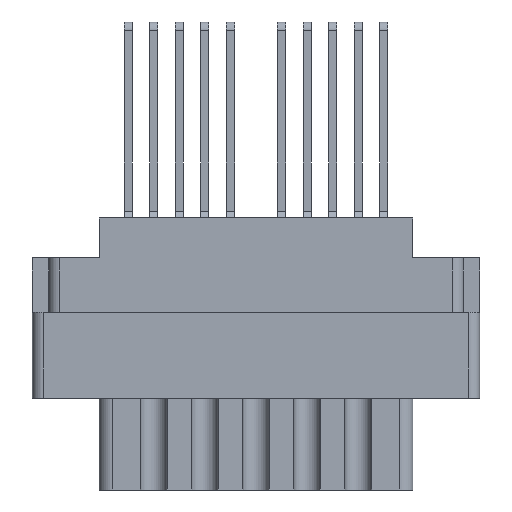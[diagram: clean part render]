
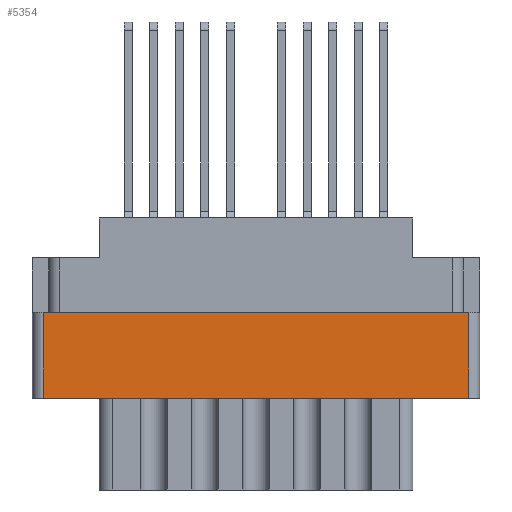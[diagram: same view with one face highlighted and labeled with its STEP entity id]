
A CAD part, front view. The second image highlights one B-rep face of the part: STEP entity #5354.
In plain terms, the highlighted planar face has unit normal (0, -1, 0).
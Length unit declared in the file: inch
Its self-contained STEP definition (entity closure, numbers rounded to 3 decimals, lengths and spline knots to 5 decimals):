
#2116 = VECTOR ( 'NONE', #2926, 39.37008 ) ;
#2384 = ORIENTED_EDGE ( 'NONE', *, *, #20708, .F. ) ;
#2432 = LINE ( 'NONE', #14155, #11054 ) ;
#2926 = DIRECTION ( 'NONE',  ( 1., 0., 0. ) ) ;
#2993 = CARTESIAN_POINT ( 'NONE',  ( -0.656, -0.343, -0.798 ) ) ;
#3983 = CARTESIAN_POINT ( 'NONE',  ( 0.624, -0.343, -0.277 ) ) ;
#5354 = ADVANCED_FACE ( 'NONE', ( #11126 ), #17944, .T. ) ;
#5846 = CARTESIAN_POINT ( 'NONE',  ( -0.624, -0.343, -0.798 ) ) ;
#7570 = ORIENTED_EDGE ( 'NONE', *, *, #15330, .F. ) ;
#8149 = VECTOR ( 'NONE', #13333, 39.37008 ) ;
#8384 = CARTESIAN_POINT ( 'NONE',  ( -0.624, -0.343, -0.529 ) ) ;
#11054 = VECTOR ( 'NONE', #14006, 39.37008 ) ;
#11126 = FACE_OUTER_BOUND ( 'NONE', #18625, .T. ) ;
#11154 = ORIENTED_EDGE ( 'NONE', *, *, #22824, .T. ) ;
#13168 = VECTOR ( 'NONE', #17793, 39.37008 ) ;
#13333 = DIRECTION ( 'NONE',  ( 0., 0., -1. ) ) ;
#13719 = LINE ( 'NONE', #5846, #8149 ) ;
#13905 = LINE ( 'NONE', #19345, #2116 ) ;
#13915 = VERTEX_POINT ( 'NONE', #3983 ) ;
#14006 = DIRECTION ( 'NONE',  ( -1., 0., 0. ) ) ;
#14082 = DIRECTION ( 'NONE',  ( 0., -1., 0. ) ) ;
#14155 = CARTESIAN_POINT ( 'NONE',  ( 0., -0.343, -0.529 ) ) ;
#14399 = CARTESIAN_POINT ( 'NONE',  ( 0.624, -0.343, -0.798 ) ) ;
#14487 = VERTEX_POINT ( 'NONE', #20200 ) ;
#15330 = EDGE_CURVE ( 'NONE', #22295, #13915, #13905, .T. ) ;
#16072 = DIRECTION ( 'NONE',  ( 0., 0., -1. ) ) ;
#16103 = CARTESIAN_POINT ( 'NONE',  ( -0.624, -0.343, -0.277 ) ) ;
#16345 = EDGE_CURVE ( 'NONE', #22295, #19529, #13719, .T. ) ;
#17549 = ORIENTED_EDGE ( 'NONE', *, *, #16345, .T. ) ;
#17793 = DIRECTION ( 'NONE',  ( 0., 0., 1. ) ) ;
#17944 = PLANE ( 'NONE',  #23078 ) ;
#18625 = EDGE_LOOP ( 'NONE', ( #7570, #17549, #2384, #11154 ) ) ;
#19345 = CARTESIAN_POINT ( 'NONE',  ( 0., -0.343, -0.277 ) ) ;
#19529 = VERTEX_POINT ( 'NONE', #8384 ) ;
#20200 = CARTESIAN_POINT ( 'NONE',  ( 0.624, -0.343, -0.529 ) ) ;
#20708 = EDGE_CURVE ( 'NONE', #14487, #19529, #2432, .T. ) ;
#22295 = VERTEX_POINT ( 'NONE', #16103 ) ;
#22716 = LINE ( 'NONE', #14399, #13168 ) ;
#22824 = EDGE_CURVE ( 'NONE', #14487, #13915, #22716, .T. ) ;
#23078 = AXIS2_PLACEMENT_3D ( 'NONE', #2993, #14082, #16072 ) ;
